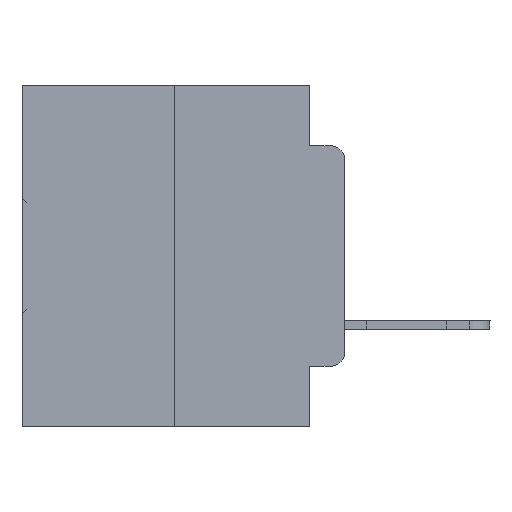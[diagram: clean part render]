
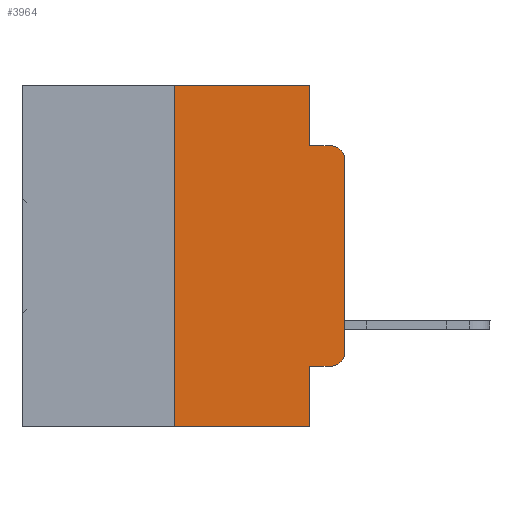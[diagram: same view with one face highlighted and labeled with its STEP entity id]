
A CAD part, left-side view. The second image highlights one B-rep face of the part: STEP entity #3964.
In plain terms, the highlighted planar face has unit normal (-1, 0, 0).
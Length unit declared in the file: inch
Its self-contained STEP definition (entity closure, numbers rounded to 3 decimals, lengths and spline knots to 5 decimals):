
#136 = ORIENTED_EDGE ( 'NONE', *, *, #5058, .T. ) ;
#367 = CARTESIAN_POINT ( 'NONE',  ( 0., 0.051, 0. ) ) ;
#452 = EDGE_CURVE ( 'NONE', #11016, #26158, #6351, .T. ) ;
#530 = EDGE_LOOP ( 'NONE', ( #136, #26407, #24543, #20287, #32062, #27672, #15594, #28066, #17614, #8706 ) ) ;
#1195 = AXIS2_PLACEMENT_3D ( 'NONE', #12642, #15279, #2437 ) ;
#1342 = FACE_OUTER_BOUND ( 'NONE', #530, .T. ) ;
#1613 = CARTESIAN_POINT ( 'NONE',  ( 0., 0., -0.1085 ) ) ;
#2437 = DIRECTION ( 'NONE',  ( 0., 0., -1. ) ) ;
#2458 = LINE ( 'NONE', #32020, #29561 ) ;
#2763 = CARTESIAN_POINT ( 'NONE',  ( 0., 0.25, -0.5 ) ) ;
#3114 = PLANE ( 'NONE',  #31904 ) ;
#3220 = DIRECTION ( 'NONE',  ( 1., 0., 0. ) ) ;
#3788 = LINE ( 'NONE', #18158, #28829 ) ;
#3964 = ADVANCED_FACE ( 'NONE', ( #1342 ), #3114, .F. ) ;
#4273 = DIRECTION ( 'NONE',  ( 0., -1., 0. ) ) ;
#5058 = EDGE_CURVE ( 'NONE', #13040, #15466, #3788, .T. ) ;
#5084 = DIRECTION ( 'NONE',  ( 0., 0., 1. ) ) ;
#6005 = VERTEX_POINT ( 'NONE', #7303 ) ;
#6326 = DIRECTION ( 'NONE',  ( 0., 0., -1. ) ) ;
#6351 = LINE ( 'NONE', #21007, #31458 ) ;
#7303 = CARTESIAN_POINT ( 'NONE',  ( 0., 0.051, -0.4115 ) ) ;
#7485 = EDGE_CURVE ( 'NONE', #15466, #31664, #20234, .T. ) ;
#8288 = CARTESIAN_POINT ( 'NONE',  ( 0., 0.473, 0. ) ) ;
#8706 = ORIENTED_EDGE ( 'NONE', *, *, #11108, .T. ) ;
#9389 = VERTEX_POINT ( 'NONE', #28228 ) ;
#9675 = EDGE_CURVE ( 'NONE', #9389, #31664, #23598, .T. ) ;
#10745 = LINE ( 'NONE', #25974, #11599 ) ;
#10882 = CARTESIAN_POINT ( 'NONE',  ( 0., 0.02, -0.0885 ) ) ;
#11016 = VERTEX_POINT ( 'NONE', #23908 ) ;
#11108 = EDGE_CURVE ( 'NONE', #31792, #13040, #16300, .T. ) ;
#11489 = EDGE_CURVE ( 'NONE', #16825, #11016, #29594, .T. ) ;
#11599 = VECTOR ( 'NONE', #30971, 39.37008 ) ;
#12642 = CARTESIAN_POINT ( 'NONE',  ( 0., 0.02, -0.1085 ) ) ;
#12650 = CARTESIAN_POINT ( 'NONE',  ( 0., 0.051, -0.0885 ) ) ;
#13040 = VERTEX_POINT ( 'NONE', #23863 ) ;
#13962 = DIRECTION ( 'NONE',  ( 0., 0., -1. ) ) ;
#13996 = EDGE_CURVE ( 'NONE', #6005, #31792, #20582, .T. ) ;
#15279 = DIRECTION ( 'NONE',  ( -1., 0., 0. ) ) ;
#15466 = VERTEX_POINT ( 'NONE', #1613 ) ;
#15594 = ORIENTED_EDGE ( 'NONE', *, *, #16708, .T. ) ;
#15886 = AXIS2_PLACEMENT_3D ( 'NONE', #16586, #19183, #6326 ) ;
#16300 = CIRCLE ( 'NONE', #15886, 0.02 ) ;
#16586 = CARTESIAN_POINT ( 'NONE',  ( 0., 0.02, -0.3915 ) ) ;
#16708 = EDGE_CURVE ( 'NONE', #16825, #25705, #2458, .T. ) ;
#16825 = VERTEX_POINT ( 'NONE', #2763 ) ;
#17125 = CARTESIAN_POINT ( 'NONE',  ( 0., 0.051, -0.5 ) ) ;
#17234 = CARTESIAN_POINT ( 'NONE',  ( 0., 0.051, -0.4115 ) ) ;
#17340 = VECTOR ( 'NONE', #4273, 39.37008 ) ;
#17614 = ORIENTED_EDGE ( 'NONE', *, *, #13996, .T. ) ;
#17930 = VECTOR ( 'NONE', #20297, 39.37008 ) ;
#18158 = CARTESIAN_POINT ( 'NONE',  ( 0., 0., 0. ) ) ;
#19183 = DIRECTION ( 'NONE',  ( -1., 0., 0. ) ) ;
#20234 = CIRCLE ( 'NONE', #1195, 0.02 ) ;
#20287 = ORIENTED_EDGE ( 'NONE', *, *, #27857, .F. ) ;
#20297 = DIRECTION ( 'NONE',  ( 0., 0., 1. ) ) ;
#20582 = LINE ( 'NONE', #17234, #17340 ) ;
#21007 = CARTESIAN_POINT ( 'NONE',  ( 0., 0.473, 0. ) ) ;
#21521 = DIRECTION ( 'NONE',  ( 0., -1., 0. ) ) ;
#22439 = LINE ( 'NONE', #26689, #28502 ) ;
#22786 = DIRECTION ( 'NONE',  ( 0., -1., 0. ) ) ;
#23598 = LINE ( 'NONE', #12650, #27241 ) ;
#23665 = DIRECTION ( 'NONE',  ( 0., -1., 0. ) ) ;
#23863 = CARTESIAN_POINT ( 'NONE',  ( 0., 0., -0.3915 ) ) ;
#23897 = DIRECTION ( 'NONE',  ( 0., 0., -1. ) ) ;
#23908 = CARTESIAN_POINT ( 'NONE',  ( 0., 0.25, 0. ) ) ;
#24543 = ORIENTED_EDGE ( 'NONE', *, *, #9675, .F. ) ;
#25705 = VERTEX_POINT ( 'NONE', #17125 ) ;
#25974 = CARTESIAN_POINT ( 'NONE',  ( 0., 0.051, 0. ) ) ;
#26158 = VERTEX_POINT ( 'NONE', #367 ) ;
#26407 = ORIENTED_EDGE ( 'NONE', *, *, #7485, .T. ) ;
#26569 = CARTESIAN_POINT ( 'NONE',  ( 0., 0.02, -0.4115 ) ) ;
#26689 = CARTESIAN_POINT ( 'NONE',  ( 0., 0.051, 0. ) ) ;
#27241 = VECTOR ( 'NONE', #22786, 39.37008 ) ;
#27672 = ORIENTED_EDGE ( 'NONE', *, *, #11489, .F. ) ;
#27857 = EDGE_CURVE ( 'NONE', #26158, #9389, #10745, .T. ) ;
#28066 = ORIENTED_EDGE ( 'NONE', *, *, #33459, .F. ) ;
#28228 = CARTESIAN_POINT ( 'NONE',  ( 0., 0.051, -0.0885 ) ) ;
#28502 = VECTOR ( 'NONE', #13962, 39.37008 ) ;
#28829 = VECTOR ( 'NONE', #5084, 39.37008 ) ;
#29561 = VECTOR ( 'NONE', #21521, 39.37008 ) ;
#29594 = LINE ( 'NONE', #33464, #17930 ) ;
#30971 = DIRECTION ( 'NONE',  ( 0., 0., -1. ) ) ;
#31458 = VECTOR ( 'NONE', #23665, 39.37008 ) ;
#31664 = VERTEX_POINT ( 'NONE', #10882 ) ;
#31792 = VERTEX_POINT ( 'NONE', #26569 ) ;
#31904 = AXIS2_PLACEMENT_3D ( 'NONE', #8288, #3220, #23897 ) ;
#32020 = CARTESIAN_POINT ( 'NONE',  ( 0., 0.473, -0.5 ) ) ;
#32062 = ORIENTED_EDGE ( 'NONE', *, *, #452, .F. ) ;
#33459 = EDGE_CURVE ( 'NONE', #6005, #25705, #22439, .T. ) ;
#33464 = CARTESIAN_POINT ( 'NONE',  ( 0., 0.25, 0. ) ) ;
